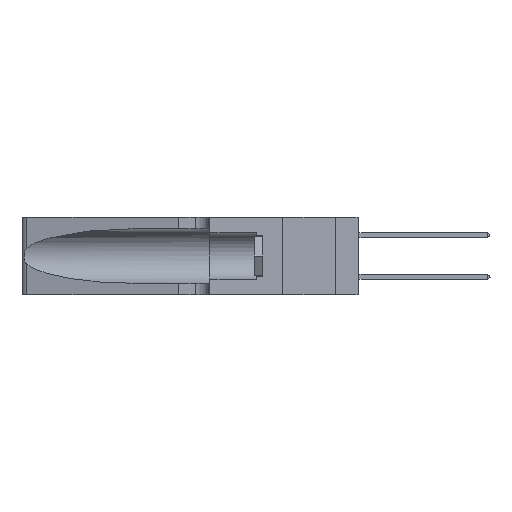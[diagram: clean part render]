
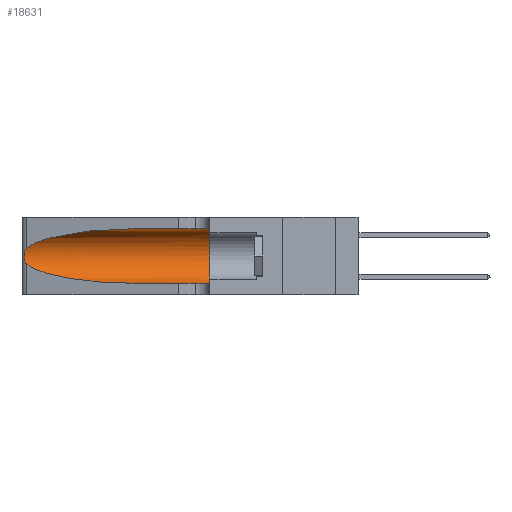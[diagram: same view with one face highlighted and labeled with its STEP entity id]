
A CAD part, left-side view. The second image highlights one B-rep face of the part: STEP entity #18631.
In plain terms, the highlighted cylindrical face has radius 3.308 mm (diameter 6.617 mm), a partial arc.
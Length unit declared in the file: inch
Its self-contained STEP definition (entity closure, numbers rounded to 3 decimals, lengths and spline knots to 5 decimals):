
#654 = ORIENTED_EDGE ( 'NONE', *, *, #20506, .T. ) ;
#1773 = CARTESIAN_POINT ( 'NONE',  ( 0.26075, 1.23896, 0.178 ) ) ;
#2221 = CARTESIAN_POINT ( 'NONE',  ( 0.2373, 1.15595, 0.28018 ) ) ;
#2572 = CARTESIAN_POINT ( 'NONE',  ( 0.1305, 0.72297, 0.31525 ) ) ;
#2957 = CARTESIAN_POINT ( 'NONE',  ( 0.25487, 1.22718, 0.14631 ) ) ;
#3189 =( BOUNDED_CURVE ( )  B_SPLINE_CURVE ( 3, ( #22348, #15795, #2221, #9037 ),
 .UNSPECIFIED., .F., .F. ) 
 B_SPLINE_CURVE_WITH_KNOTS ( ( 4, 4 ),
 ( 1.5708, 2.84003 ),
 .UNSPECIFIED. ) 
 CURVE ( )  GEOMETRIC_REPRESENTATION_ITEM ( )  RATIONAL_B_SPLINE_CURVE ( ( 1., 0.87, 0.87, 1. ) ) 
 REPRESENTATION_ITEM ( '' )  );
#3525 = FACE_OUTER_BOUND ( 'NONE', #20345, .T. ) ;
#3532 = ORIENTED_EDGE ( 'NONE', *, *, #16453, .T. ) ;
#3616 = CARTESIAN_POINT ( 'NONE',  ( 0.26017, 1.23833, 0.17102 ) ) ;
#4988 = ORIENTED_EDGE ( 'NONE', *, *, #12732, .T. ) ;
#5300 = EDGE_CURVE ( 'NONE', #6755, #19560, #24509, .T. ) ;
#5776 = DIRECTION ( 'NONE',  ( 0., 0., 1. ) ) ;
#6042 = CARTESIAN_POINT ( 'NONE',  ( 0.25854, 1.2359, 0.20912 ) ) ;
#6741 = VECTOR ( 'NONE', #19939, 39.37008 ) ;
#6755 = VERTEX_POINT ( 'NONE', #2572 ) ;
#7499 = VECTOR ( 'NONE', #22835, 39.37008 ) ;
#8194 = CARTESIAN_POINT ( 'NONE',  ( 0.25787, 1.23484, 0.2124 ) ) ;
#8317 = VERTEX_POINT ( 'NONE', #21518 ) ;
#9037 = CARTESIAN_POINT ( 'NONE',  ( 0.25487, 1.22718, 0.22369 ) ) ;
#9170 = ORIENTED_EDGE ( 'NONE', *, *, #9456, .T. ) ;
#9239 = LINE ( 'NONE', #20421, #7499 ) ;
#9456 = EDGE_CURVE ( 'NONE', #20191, #14638, #24764, .T. ) ;
#10307 = DIRECTION ( 'NONE',  ( 0., -1., 0. ) ) ;
#10439 = CIRCLE ( 'NONE', #19839, 0.13025 ) ;
#11927 = ORIENTED_EDGE ( 'NONE', *, *, #5300, .F. ) ;
#12449 = CARTESIAN_POINT ( 'NONE',  ( 0.25639, 1.23186, 0.15144 ) ) ;
#12645 = CARTESIAN_POINT ( 'NONE',  ( 0.25789, 1.23486, 0.15765 ) ) ;
#12732 = EDGE_CURVE ( 'NONE', #6755, #21892, #3189, .T. ) ;
#13308 = CARTESIAN_POINT ( 'NONE',  ( 0.1305, 1.61858, 0.31525 ) ) ;
#14568 = DIRECTION ( 'NONE',  ( 0., 0., -1. ) ) ;
#14638 = VERTEX_POINT ( 'NONE', #16056 ) ;
#14891 = CARTESIAN_POINT ( 'NONE',  ( 0.1305, 0.35, 0.185 ) ) ;
#14961 = CARTESIAN_POINT ( 'NONE',  ( 0.25487, 1.22718, 0.22369 ) ) ;
#15513 = AXIS2_PLACEMENT_3D ( 'NONE', #25697, #10307, #14568 ) ;
#15795 = CARTESIAN_POINT ( 'NONE',  ( 0.18966, 0.96281, 0.31525 ) ) ;
#15973 = CARTESIAN_POINT ( 'NONE',  ( 0.25487, 1.22718, 0.14631 ) ) ;
#16056 = CARTESIAN_POINT ( 'NONE',  ( 0.1305, 0.72297, 0.05475 ) ) ;
#16453 = EDGE_CURVE ( 'NONE', #14638, #8317, #9239, .T. ) ;
#17411 = CYLINDRICAL_SURFACE ( 'NONE', #15513, 0.13025 ) ;
#18027 = ORIENTED_EDGE ( 'NONE', *, *, #19791, .F. ) ;
#18631 = ADVANCED_FACE ( 'NONE', ( #3525 ), #17411, .F. ) ;
#19095 = DIRECTION ( 'NONE',  ( 0., 1., 0. ) ) ;
#19560 = VERTEX_POINT ( 'NONE', #22901 ) ;
#19567 = CARTESIAN_POINT ( 'NONE',  ( 0.25555, 1.22994, 0.2215 ) ) ;
#19791 = EDGE_CURVE ( 'NONE', #19560, #8317, #10439, .T. ) ;
#19839 = AXIS2_PLACEMENT_3D ( 'NONE', #14891, #19095, #5776 ) ;
#19939 = DIRECTION ( 'NONE',  ( 0., -1., 0. ) ) ;
#20191 = VERTEX_POINT ( 'NONE', #2957 ) ;
#20345 = EDGE_LOOP ( 'NONE', ( #4988, #654, #9170, #3532, #18027, #11927 ) ) ;
#20421 = CARTESIAN_POINT ( 'NONE',  ( 0.1305, 1.61858, 0.05475 ) ) ;
#20506 = EDGE_CURVE ( 'NONE', #21892, #20191, #21720, .T. ) ;
#21518 = CARTESIAN_POINT ( 'NONE',  ( 0.1305, 0.35, 0.05475 ) ) ;
#21720 = B_SPLINE_CURVE_WITH_KNOTS ( 'NONE', 3,
 ( #14961, #19567, #28322, #8194, #6042, #28422, #23739, #1773, #3616, #23840, #12645, #12449, #25989, #28120 ),
 .UNSPECIFIED., .F., .F.,
 ( 4, 2, 2, 2, 2, 2, 4 ),
 ( 0., 0.00027, 0.00053, 0.00107, 0.0016, 0.00187, 0.00214 ),
 .UNSPECIFIED. ) ;
#21892 = VERTEX_POINT ( 'NONE', #28718 ) ;
#22348 = CARTESIAN_POINT ( 'NONE',  ( 0.1305, 0.72297, 0.31525 ) ) ;
#22701 = CARTESIAN_POINT ( 'NONE',  ( 0.18966, 0.96281, 0.05475 ) ) ;
#22835 = DIRECTION ( 'NONE',  ( 0., -1., 0. ) ) ;
#22901 = CARTESIAN_POINT ( 'NONE',  ( 0.1305, 0.35, 0.31525 ) ) ;
#23739 = CARTESIAN_POINT ( 'NONE',  ( 0.26075, 1.23896, 0.19203 ) ) ;
#23840 = CARTESIAN_POINT ( 'NONE',  ( 0.25856, 1.23593, 0.16098 ) ) ;
#24509 = LINE ( 'NONE', #13308, #6741 ) ;
#24764 =( BOUNDED_CURVE ( )  B_SPLINE_CURVE ( 3, ( #15973, #27195, #22701, #27570 ),
 .UNSPECIFIED., .F., .F. ) 
 B_SPLINE_CURVE_WITH_KNOTS ( ( 4, 4 ),
 ( 3.44316, 4.71239 ),
 .UNSPECIFIED. ) 
 CURVE ( )  GEOMETRIC_REPRESENTATION_ITEM ( )  RATIONAL_B_SPLINE_CURVE ( ( 1., 0.87, 0.87, 1. ) ) 
 REPRESENTATION_ITEM ( '' )  );
#25697 = CARTESIAN_POINT ( 'NONE',  ( 0.1305, 1.61858, 0.185 ) ) ;
#25989 = CARTESIAN_POINT ( 'NONE',  ( 0.25555, 1.22993, 0.14849 ) ) ;
#27195 = CARTESIAN_POINT ( 'NONE',  ( 0.2373, 1.15595, 0.08982 ) ) ;
#27570 = CARTESIAN_POINT ( 'NONE',  ( 0.1305, 0.72297, 0.05475 ) ) ;
#28120 = CARTESIAN_POINT ( 'NONE',  ( 0.25487, 1.22718, 0.14631 ) ) ;
#28322 = CARTESIAN_POINT ( 'NONE',  ( 0.25639, 1.23184, 0.21858 ) ) ;
#28422 = CARTESIAN_POINT ( 'NONE',  ( 0.26018, 1.23835, 0.19895 ) ) ;
#28718 = CARTESIAN_POINT ( 'NONE',  ( 0.25487, 1.22718, 0.22369 ) ) ;
